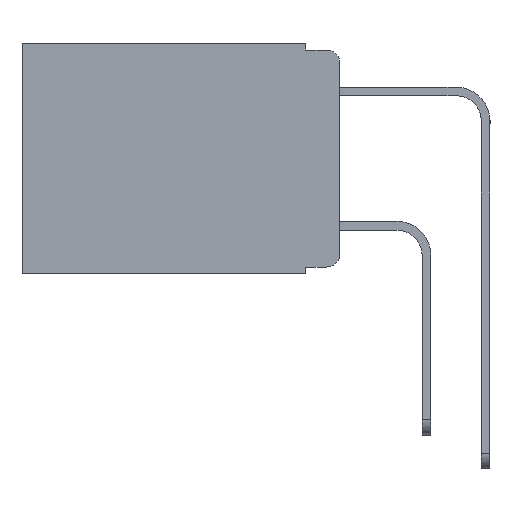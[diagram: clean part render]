
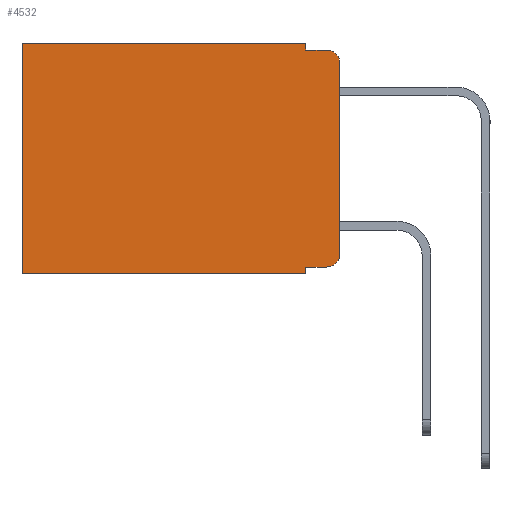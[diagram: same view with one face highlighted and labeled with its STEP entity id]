
A CAD part, left-side view. The second image highlights one B-rep face of the part: STEP entity #4532.
In plain terms, the highlighted planar face has unit normal (-1, 0, 0).
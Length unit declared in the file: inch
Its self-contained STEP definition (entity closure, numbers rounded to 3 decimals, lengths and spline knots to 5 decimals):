
#594 = VECTOR ( 'NONE', #1575, 39.37008 ) ;
#952 = LINE ( 'NONE', #6743, #9474 ) ;
#1048 = EDGE_CURVE ( 'NONE', #11440, #9336, #7396, .T. ) ;
#1479 = VERTEX_POINT ( 'NONE', #8477 ) ;
#1575 = DIRECTION ( 'NONE',  ( 0., 0., -1. ) ) ;
#1716 = DIRECTION ( 'NONE',  ( 0., 0., -1. ) ) ;
#2281 = DIRECTION ( 'NONE',  ( 0., 1., 0. ) ) ;
#2373 = CARTESIAN_POINT ( 'NONE',  ( 0.298, 0., -0.343 ) ) ;
#3153 = CARTESIAN_POINT ( 'NONE',  ( 0.298, 0.02, -0.01 ) ) ;
#3164 = EDGE_CURVE ( 'NONE', #9336, #10220, #5790, .T. ) ;
#4216 = EDGE_CURVE ( 'NONE', #1479, #10220, #17644, .T. ) ;
#4433 = VECTOR ( 'NONE', #2281, 39.37008 ) ;
#4532 = ADVANCED_FACE ( 'NONE', ( #12775 ), #14906, .F. ) ;
#4805 = DIRECTION ( 'NONE',  ( 0., -1., 0. ) ) ;
#5360 = CIRCLE ( 'NONE', #20145, 0.02 ) ;
#5790 = LINE ( 'NONE', #15983, #9069 ) ;
#5979 = ORIENTED_EDGE ( 'NONE', *, *, #15352, .T. ) ;
#5980 = CARTESIAN_POINT ( 'NONE',  ( 0.298, 0.473, 0. ) ) ;
#6084 = CARTESIAN_POINT ( 'NONE',  ( 0.298, 0., -0.313 ) ) ;
#6563 = DIRECTION ( 'NONE',  ( -1., 0., 0. ) ) ;
#6602 = VECTOR ( 'NONE', #7597, 39.37008 ) ;
#6743 = CARTESIAN_POINT ( 'NONE',  ( 0.298, 0.051, 0. ) ) ;
#6901 = VECTOR ( 'NONE', #1716, 39.37008 ) ;
#6945 = LINE ( 'NONE', #5980, #18970 ) ;
#7396 = LINE ( 'NONE', #8489, #6901 ) ;
#7521 = ORIENTED_EDGE ( 'NONE', *, *, #10480, .T. ) ;
#7536 = EDGE_CURVE ( 'NONE', #1479, #9408, #13402, .T. ) ;
#7597 = DIRECTION ( 'NONE',  ( 0., -1., 0. ) ) ;
#8477 = CARTESIAN_POINT ( 'NONE',  ( 0.298, 0., -0.03 ) ) ;
#8489 = CARTESIAN_POINT ( 'NONE',  ( 0.298, 0.051, 0. ) ) ;
#9069 = VECTOR ( 'NONE', #4805, 39.37008 ) ;
#9336 = VERTEX_POINT ( 'NONE', #16987 ) ;
#9408 = VERTEX_POINT ( 'NONE', #6084 ) ;
#9417 = DIRECTION ( 'NONE',  ( -1., 0., 0. ) ) ;
#9438 = CARTESIAN_POINT ( 'NONE',  ( 0.298, 0.473, -0.343 ) ) ;
#9474 = VECTOR ( 'NONE', #17770, 39.37008 ) ;
#9500 = VERTEX_POINT ( 'NONE', #9438 ) ;
#9745 = ORIENTED_EDGE ( 'NONE', *, *, #16415, .T. ) ;
#9827 = VERTEX_POINT ( 'NONE', #11925 ) ;
#10209 = DIRECTION ( 'NONE',  ( 0., 0., -1. ) ) ;
#10220 = VERTEX_POINT ( 'NONE', #3153 ) ;
#10261 = ORIENTED_EDGE ( 'NONE', *, *, #18439, .F. ) ;
#10480 = EDGE_CURVE ( 'NONE', #11440, #9827, #20231, .T. ) ;
#10574 = CARTESIAN_POINT ( 'NONE',  ( 0.298, 0.051, -0.343 ) ) ;
#10647 = LINE ( 'NONE', #2373, #17529 ) ;
#10809 = VERTEX_POINT ( 'NONE', #20367 ) ;
#10814 = DIRECTION ( 'NONE',  ( 0., 0., -1. ) ) ;
#10843 = LINE ( 'NONE', #20026, #6602 ) ;
#11198 = CARTESIAN_POINT ( 'NONE',  ( 0.298, 0., 0. ) ) ;
#11434 = VERTEX_POINT ( 'NONE', #17451 ) ;
#11440 = VERTEX_POINT ( 'NONE', #20478 ) ;
#11758 = ORIENTED_EDGE ( 'NONE', *, *, #7536, .F. ) ;
#11904 = CARTESIAN_POINT ( 'NONE',  ( 0.298, 0., 0. ) ) ;
#11925 = CARTESIAN_POINT ( 'NONE',  ( 0.298, 0.473, 0. ) ) ;
#11999 = DIRECTION ( 'NONE',  ( 0., 1., 0. ) ) ;
#12001 = ORIENTED_EDGE ( 'NONE', *, *, #3164, .F. ) ;
#12775 = FACE_OUTER_BOUND ( 'NONE', #17139, .T. ) ;
#13402 = LINE ( 'NONE', #11198, #594 ) ;
#14473 = AXIS2_PLACEMENT_3D ( 'NONE', #18810, #9417, #20334 ) ;
#14906 = PLANE ( 'NONE',  #19248 ) ;
#14957 = ORIENTED_EDGE ( 'NONE', *, *, #20464, .T. ) ;
#15352 = EDGE_CURVE ( 'NONE', #10809, #9408, #5360, .T. ) ;
#15658 = ORIENTED_EDGE ( 'NONE', *, *, #1048, .F. ) ;
#15983 = CARTESIAN_POINT ( 'NONE',  ( 0.298, 0.051, -0.01 ) ) ;
#16072 = CARTESIAN_POINT ( 'NONE',  ( 0.298, 0.02, -0.313 ) ) ;
#16333 = VERTEX_POINT ( 'NONE', #10574 ) ;
#16415 = EDGE_CURVE ( 'NONE', #11434, #10809, #10843, .T. ) ;
#16987 = CARTESIAN_POINT ( 'NONE',  ( 0.298, 0.051, -0.01 ) ) ;
#17139 = EDGE_LOOP ( 'NONE', ( #11758, #19510, #12001, #15658, #7521, #14957, #18568, #10261, #9745, #5979 ) ) ;
#17451 = CARTESIAN_POINT ( 'NONE',  ( 0.298, 0.051, -0.333 ) ) ;
#17529 = VECTOR ( 'NONE', #11999, 39.37008 ) ;
#17612 = DIRECTION ( 'NONE',  ( 0., 0., -1. ) ) ;
#17644 = CIRCLE ( 'NONE', #14473, 0.02 ) ;
#17770 = DIRECTION ( 'NONE',  ( 0., 0., -1. ) ) ;
#18012 = CARTESIAN_POINT ( 'NONE',  ( 0.298, 0., 0. ) ) ;
#18439 = EDGE_CURVE ( 'NONE', #11434, #16333, #952, .T. ) ;
#18568 = ORIENTED_EDGE ( 'NONE', *, *, #20355, .F. ) ;
#18810 = CARTESIAN_POINT ( 'NONE',  ( 0.298, 0.02, -0.03 ) ) ;
#18970 = VECTOR ( 'NONE', #10814, 39.37008 ) ;
#19248 = AXIS2_PLACEMENT_3D ( 'NONE', #18012, #19546, #10209 ) ;
#19510 = ORIENTED_EDGE ( 'NONE', *, *, #4216, .T. ) ;
#19546 = DIRECTION ( 'NONE',  ( 1., 0., 0. ) ) ;
#20026 = CARTESIAN_POINT ( 'NONE',  ( 0.298, 0.051, -0.333 ) ) ;
#20145 = AXIS2_PLACEMENT_3D ( 'NONE', #16072, #6563, #17612 ) ;
#20231 = LINE ( 'NONE', #11904, #4433 ) ;
#20334 = DIRECTION ( 'NONE',  ( 0., 0., -1. ) ) ;
#20355 = EDGE_CURVE ( 'NONE', #16333, #9500, #10647, .T. ) ;
#20367 = CARTESIAN_POINT ( 'NONE',  ( 0.298, 0.02, -0.333 ) ) ;
#20464 = EDGE_CURVE ( 'NONE', #9827, #9500, #6945, .T. ) ;
#20478 = CARTESIAN_POINT ( 'NONE',  ( 0.298, 0.051, 0. ) ) ;
